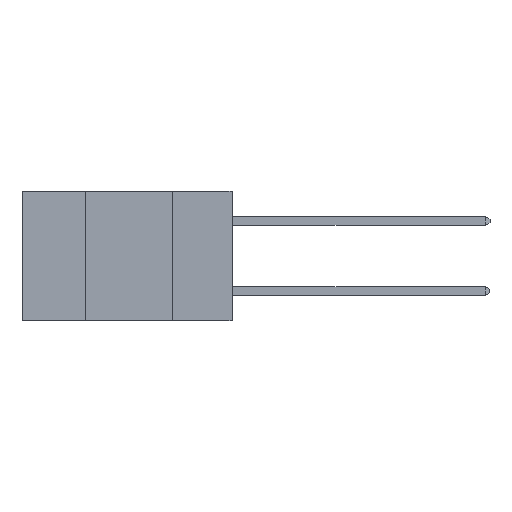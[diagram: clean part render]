
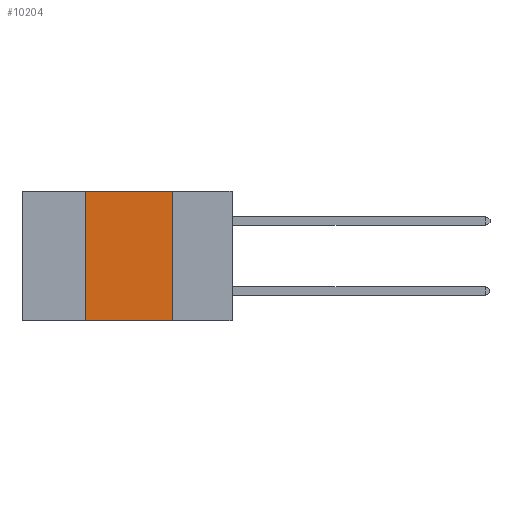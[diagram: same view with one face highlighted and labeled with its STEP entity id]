
A CAD part, left-side view. The second image highlights one B-rep face of the part: STEP entity #10204.
In plain terms, the highlighted planar face has unit normal (-1, 0, 0).
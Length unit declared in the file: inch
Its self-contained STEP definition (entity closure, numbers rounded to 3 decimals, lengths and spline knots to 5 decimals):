
#893 = VERTEX_POINT ( 'NONE', #9766 ) ;
#1714 = LINE ( 'NONE', #8780, #8438 ) ;
#2286 = VECTOR ( 'NONE', #10578, 39.37008 ) ;
#2506 = EDGE_LOOP ( 'NONE', ( #8241, #11091, #6041, #3084 ) ) ;
#2948 = VERTEX_POINT ( 'NONE', #8575 ) ;
#3084 = ORIENTED_EDGE ( 'NONE', *, *, #6239, .T. ) ;
#3563 = DIRECTION ( 'NONE',  ( 0., 0., 1. ) ) ;
#3843 = VECTOR ( 'NONE', #7771, 39.37008 ) ;
#3930 = CARTESIAN_POINT ( 'NONE',  ( 0., 0.6, 0. ) ) ;
#4061 = VERTEX_POINT ( 'NONE', #6583 ) ;
#4110 = LINE ( 'NONE', #8672, #3843 ) ;
#4650 = VECTOR ( 'NONE', #10027, 39.37008 ) ;
#4973 = VERTEX_POINT ( 'NONE', #11236 ) ;
#5088 = CARTESIAN_POINT ( 'NONE',  ( 0., 0.6, 0. ) ) ;
#5948 = DIRECTION ( 'NONE',  ( 0., 0., -1. ) ) ;
#6041 = ORIENTED_EDGE ( 'NONE', *, *, #8227, .F. ) ;
#6239 = EDGE_CURVE ( 'NONE', #4061, #2948, #4110, .T. ) ;
#6583 = CARTESIAN_POINT ( 'NONE',  ( 0., 0.42, -0.37 ) ) ;
#6598 = EDGE_CURVE ( 'NONE', #4973, #893, #6949, .T. ) ;
#6906 = AXIS2_PLACEMENT_3D ( 'NONE', #5088, #11154, #5948 ) ;
#6949 = LINE ( 'NONE', #3930, #4650 ) ;
#7044 = EDGE_CURVE ( 'NONE', #893, #2948, #9272, .T. ) ;
#7771 = DIRECTION ( 'NONE',  ( 0., -1., 0. ) ) ;
#8227 = EDGE_CURVE ( 'NONE', #4061, #4973, #1714, .T. ) ;
#8241 = ORIENTED_EDGE ( 'NONE', *, *, #7044, .F. ) ;
#8438 = VECTOR ( 'NONE', #3563, 39.37008 ) ;
#8537 = FACE_OUTER_BOUND ( 'NONE', #2506, .T. ) ;
#8575 = CARTESIAN_POINT ( 'NONE',  ( 0., 0.17, -0.37 ) ) ;
#8672 = CARTESIAN_POINT ( 'NONE',  ( 0., 0.6, -0.37 ) ) ;
#8780 = CARTESIAN_POINT ( 'NONE',  ( 0., 0.42, 0. ) ) ;
#8836 = CARTESIAN_POINT ( 'NONE',  ( 0., 0.17, 0. ) ) ;
#9272 = LINE ( 'NONE', #8836, #2286 ) ;
#9424 = PLANE ( 'NONE',  #6906 ) ;
#9766 = CARTESIAN_POINT ( 'NONE',  ( 0., 0.17, 0. ) ) ;
#10027 = DIRECTION ( 'NONE',  ( 0., -1., 0. ) ) ;
#10204 = ADVANCED_FACE ( 'NONE', ( #8537 ), #9424, .F. ) ;
#10578 = DIRECTION ( 'NONE',  ( 0., 0., -1. ) ) ;
#11091 = ORIENTED_EDGE ( 'NONE', *, *, #6598, .F. ) ;
#11154 = DIRECTION ( 'NONE',  ( 1., 0., 0. ) ) ;
#11236 = CARTESIAN_POINT ( 'NONE',  ( 0., 0.42, 0. ) ) ;
